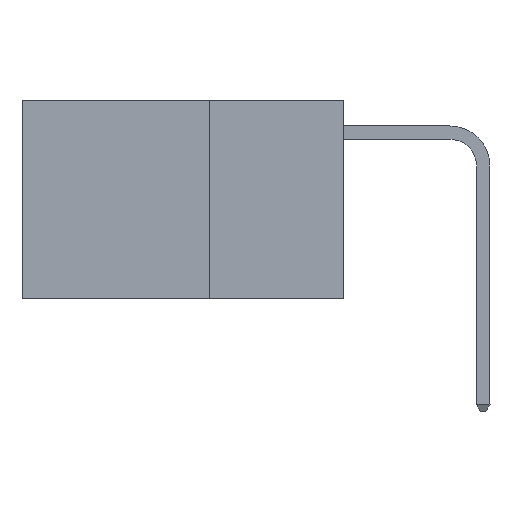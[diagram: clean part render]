
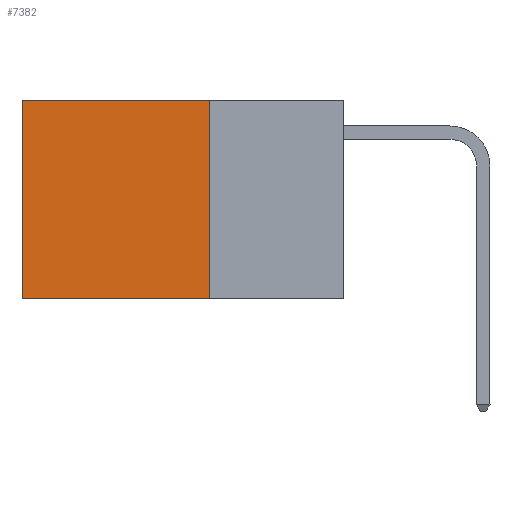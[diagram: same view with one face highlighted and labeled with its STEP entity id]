
A CAD part, left-side view. The second image highlights one B-rep face of the part: STEP entity #7382.
In plain terms, the highlighted planar face has unit normal (-1, 0, 0).
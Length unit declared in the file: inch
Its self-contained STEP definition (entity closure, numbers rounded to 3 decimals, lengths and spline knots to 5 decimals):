
#40 = CARTESIAN_POINT ( 'NONE',  ( 0.2625, 0.25, 0. ) ) ;
#66 = ORIENTED_EDGE ( 'NONE', *, *, #6228, .F. ) ;
#186 = PLANE ( 'NONE',  #17705 ) ;
#1137 = DIRECTION ( 'NONE',  ( 0., 0., -1. ) ) ;
#1196 = CARTESIAN_POINT ( 'NONE',  ( 0.2625, 0.25, 0. ) ) ;
#1265 = VECTOR ( 'NONE', #1475, 39.37008 ) ;
#1475 = DIRECTION ( 'NONE',  ( 0., 0., -1. ) ) ;
#1482 = ORIENTED_EDGE ( 'NONE', *, *, #17512, .T. ) ;
#1950 = ORIENTED_EDGE ( 'NONE', *, *, #18024, .F. ) ;
#5328 = FACE_OUTER_BOUND ( 'NONE', #11960, .T. ) ;
#5615 = DIRECTION ( 'NONE',  ( 0., 1., 0. ) ) ;
#6181 = CARTESIAN_POINT ( 'NONE',  ( 0.2625, 0.6, 0. ) ) ;
#6228 = EDGE_CURVE ( 'NONE', #8148, #12431, #13842, .T. ) ;
#6805 = VERTEX_POINT ( 'NONE', #6181 ) ;
#7382 = ADVANCED_FACE ( 'NONE', ( #5328 ), #186, .F. ) ;
#8148 = VERTEX_POINT ( 'NONE', #18454 ) ;
#10396 = CARTESIAN_POINT ( 'NONE',  ( 0.2625, 0.25, -0.37 ) ) ;
#11046 = LINE ( 'NONE', #18354, #18598 ) ;
#11960 = EDGE_LOOP ( 'NONE', ( #1482, #1950, #66, #12482 ) ) ;
#12431 = VERTEX_POINT ( 'NONE', #10396 ) ;
#12482 = ORIENTED_EDGE ( 'NONE', *, *, #17394, .T. ) ;
#12752 = DIRECTION ( 'NONE',  ( 0., 1., 0. ) ) ;
#13824 = VECTOR ( 'NONE', #1137, 39.37008 ) ;
#13842 = LINE ( 'NONE', #1196, #13824 ) ;
#15111 = LINE ( 'NONE', #18520, #17918 ) ;
#16002 = VERTEX_POINT ( 'NONE', #18376 ) ;
#16432 = LINE ( 'NONE', #18827, #1265 ) ;
#17394 = EDGE_CURVE ( 'NONE', #8148, #6805, #11046, .T. ) ;
#17512 = EDGE_CURVE ( 'NONE', #6805, #16002, #16432, .T. ) ;
#17705 = AXIS2_PLACEMENT_3D ( 'NONE', #40, #18462, #18278 ) ;
#17918 = VECTOR ( 'NONE', #5615, 39.37008 ) ;
#18024 = EDGE_CURVE ( 'NONE', #12431, #16002, #15111, .T. ) ;
#18278 = DIRECTION ( 'NONE',  ( 0., 0., -1. ) ) ;
#18354 = CARTESIAN_POINT ( 'NONE',  ( 0.2625, 0.25, 0. ) ) ;
#18376 = CARTESIAN_POINT ( 'NONE',  ( 0.2625, 0.6, -0.37 ) ) ;
#18454 = CARTESIAN_POINT ( 'NONE',  ( 0.2625, 0.25, 0. ) ) ;
#18462 = DIRECTION ( 'NONE',  ( 1., 0., 0. ) ) ;
#18520 = CARTESIAN_POINT ( 'NONE',  ( 0.2625, 0.25, -0.37 ) ) ;
#18598 = VECTOR ( 'NONE', #12752, 39.37008 ) ;
#18827 = CARTESIAN_POINT ( 'NONE',  ( 0.2625, 0.6, 0. ) ) ;
